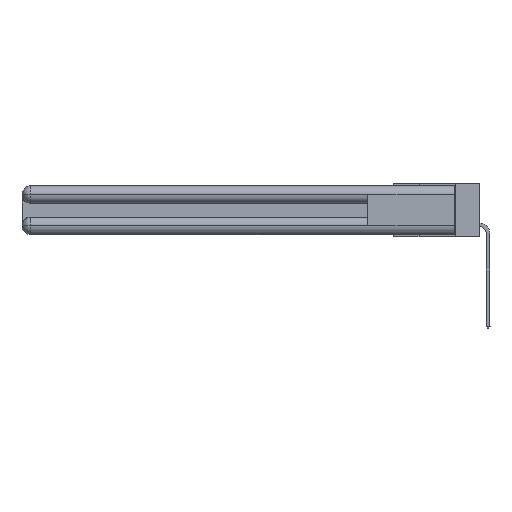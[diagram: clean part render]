
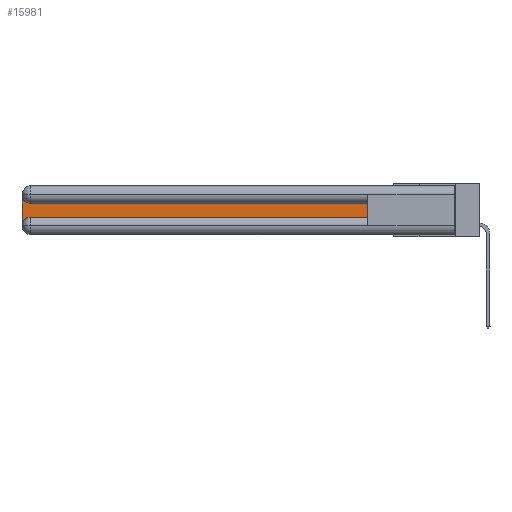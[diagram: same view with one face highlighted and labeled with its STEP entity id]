
A CAD part, left-side view. The second image highlights one B-rep face of the part: STEP entity #15981.
In plain terms, the highlighted planar face has unit normal (-1, 0, 0).
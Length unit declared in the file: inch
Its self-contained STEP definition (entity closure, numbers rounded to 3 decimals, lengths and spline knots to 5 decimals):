
#31 = CARTESIAN_POINT ( 'NONE',  ( 0.075, 3., -0.2175 ) ) ;
#1408 = ORIENTED_EDGE ( 'NONE', *, *, #21222, .T. ) ;
#1516 = CARTESIAN_POINT ( 'NONE',  ( 0.075, 0.6, -0.2175 ) ) ;
#1831 = ORIENTED_EDGE ( 'NONE', *, *, #21924, .T. ) ;
#2036 = DIRECTION ( 'NONE',  ( 0., 0., -1. ) ) ;
#2083 = CARTESIAN_POINT ( 'NONE',  ( 0.075, 3., -0.1225 ) ) ;
#3097 = ORIENTED_EDGE ( 'NONE', *, *, #6496, .T. ) ;
#4640 = VERTEX_POINT ( 'NONE', #27968 ) ;
#5208 = DIRECTION ( 'NONE',  ( 1., 0., 0. ) ) ;
#5685 = CARTESIAN_POINT ( 'NONE',  ( 0.075, 2.94, -0.1225 ) ) ;
#6366 = DIRECTION ( 'NONE',  ( 0., 0., 1. ) ) ;
#6496 = EDGE_CURVE ( 'NONE', #22079, #4640, #17982, .T. ) ;
#6505 = CARTESIAN_POINT ( 'NONE',  ( 0.075, 0.6, -0.1225 ) ) ;
#7056 = LINE ( 'NONE', #6505, #26344 ) ;
#7298 = DIRECTION ( 'NONE',  ( 1., 0., 0. ) ) ;
#7500 = CARTESIAN_POINT ( 'NONE',  ( 0.075, 3., -0.0625 ) ) ;
#7544 = CARTESIAN_POINT ( 'NONE',  ( 0.075, 2.94, -0.0625 ) ) ;
#7760 = AXIS2_PLACEMENT_3D ( 'NONE', #2083, #23502, #9807 ) ;
#7886 = DIRECTION ( 'NONE',  ( 0., 0., -1. ) ) ;
#8230 = CARTESIAN_POINT ( 'NONE',  ( 0.075, 0.6, -0.2175 ) ) ;
#8929 = CARTESIAN_POINT ( 'NONE',  ( 0.075, 0.6, -0.2175 ) ) ;
#9185 = ORIENTED_EDGE ( 'NONE', *, *, #32668, .T. ) ;
#9807 = DIRECTION ( 'NONE',  ( 0., 0., -1. ) ) ;
#9856 = AXIS2_PLACEMENT_3D ( 'NONE', #23335, #7298, #2036 ) ;
#10256 = CIRCLE ( 'NONE', #31056, 0.06 ) ;
#11048 = CARTESIAN_POINT ( 'NONE',  ( 0.075, 2.94, -0.2175 ) ) ;
#11725 = DIRECTION ( 'NONE',  ( 0., 0., -1. ) ) ;
#12625 = EDGE_CURVE ( 'NONE', #20877, #22220, #10256, .T. ) ;
#13495 = DIRECTION ( 'NONE',  ( 0., -1., 0. ) ) ;
#15230 = ORIENTED_EDGE ( 'NONE', *, *, #12625, .T. ) ;
#15981 = ADVANCED_FACE ( 'NONE', ( #27557 ), #25727, .F. ) ;
#16736 = VECTOR ( 'NONE', #6366, 39.37008 ) ;
#16937 = CARTESIAN_POINT ( 'NONE',  ( 0.075, 3., -0.2775 ) ) ;
#17792 = VERTEX_POINT ( 'NONE', #11048 ) ;
#17982 = LINE ( 'NONE', #8929, #16736 ) ;
#19373 = DIRECTION ( 'NONE',  ( 0., 1., 0. ) ) ;
#20452 = LINE ( 'NONE', #31, #23349 ) ;
#20877 = VERTEX_POINT ( 'NONE', #5685 ) ;
#21222 = EDGE_CURVE ( 'NONE', #30466, #17792, #25057, .T. ) ;
#21924 = EDGE_CURVE ( 'NONE', #22220, #30466, #20452, .T. ) ;
#22079 = VERTEX_POINT ( 'NONE', #1516 ) ;
#22220 = VERTEX_POINT ( 'NONE', #7500 ) ;
#23335 = CARTESIAN_POINT ( 'NONE',  ( 0.075, 2.94, -0.2775 ) ) ;
#23349 = VECTOR ( 'NONE', #11725, 39.37008 ) ;
#23423 = EDGE_CURVE ( 'NONE', #17792, #22079, #33968, .T. ) ;
#23502 = DIRECTION ( 'NONE',  ( 1., 0., 0. ) ) ;
#25057 = CIRCLE ( 'NONE', #9856, 0.06 ) ;
#25727 = PLANE ( 'NONE',  #7760 ) ;
#26344 = VECTOR ( 'NONE', #19373, 39.37008 ) ;
#27557 = FACE_OUTER_BOUND ( 'NONE', #31833, .T. ) ;
#27968 = CARTESIAN_POINT ( 'NONE',  ( 0.075, 0.6, -0.1225 ) ) ;
#28076 = ORIENTED_EDGE ( 'NONE', *, *, #23423, .T. ) ;
#30466 = VERTEX_POINT ( 'NONE', #16937 ) ;
#31056 = AXIS2_PLACEMENT_3D ( 'NONE', #7544, #5208, #7886 ) ;
#31833 = EDGE_LOOP ( 'NONE', ( #9185, #15230, #1831, #1408, #28076, #3097 ) ) ;
#32668 = EDGE_CURVE ( 'NONE', #4640, #20877, #7056, .T. ) ;
#33522 = VECTOR ( 'NONE', #13495, 39.37008 ) ;
#33968 = LINE ( 'NONE', #8230, #33522 ) ;
